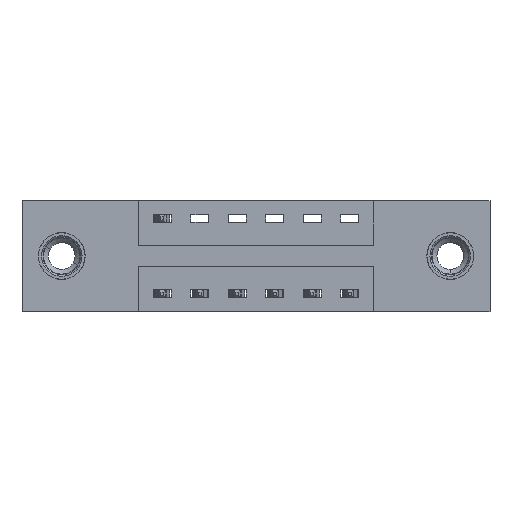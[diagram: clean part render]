
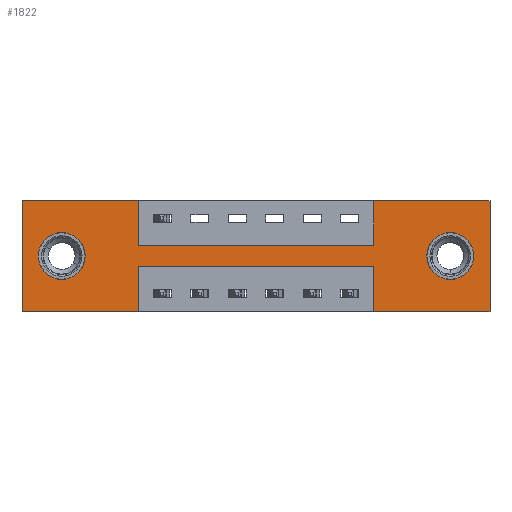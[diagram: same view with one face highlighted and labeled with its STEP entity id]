
A CAD part, front view. The second image highlights one B-rep face of the part: STEP entity #1822.
In plain terms, the highlighted planar face has unit normal (0, -1, 0).
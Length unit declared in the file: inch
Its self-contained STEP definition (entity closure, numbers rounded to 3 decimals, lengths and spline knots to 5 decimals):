
#137 = EDGE_CURVE ( 'NONE', #8113, #5049, #6763, .T. ) ;
#232 = DIRECTION ( 'NONE',  ( 0., 1., 0. ) ) ;
#270 = FACE_BOUND ( 'NONE', #4870, .T. ) ;
#615 = CARTESIAN_POINT ( 'NONE',  ( 0.3875, 0., 0. ) ) ;
#638 = EDGE_CURVE ( 'NONE', #8432, #5361, #3279, .T. ) ;
#784 = CIRCLE ( 'NONE', #4674, 0.078 ) ;
#791 = CARTESIAN_POINT ( 'NONE',  ( 0., 0., 0. ) ) ;
#846 = VERTEX_POINT ( 'NONE', #2154 ) ;
#847 = ORIENTED_EDGE ( 'NONE', *, *, #6527, .T. ) ;
#1048 = EDGE_CURVE ( 'NONE', #5049, #8432, #7312, .T. ) ;
#1092 = CARTESIAN_POINT ( 'NONE',  ( 1.1725, 0., -0.37 ) ) ;
#1111 = CARTESIAN_POINT ( 'NONE',  ( 0.1325, 0., -0.263 ) ) ;
#1154 = EDGE_CURVE ( 'NONE', #3479, #5919, #2931, .T. ) ;
#1217 = LINE ( 'NONE', #3399, #6909 ) ;
#1261 = VECTOR ( 'NONE', #5626, 39.37008 ) ;
#1312 = ORIENTED_EDGE ( 'NONE', *, *, #8654, .F. ) ;
#1360 = ORIENTED_EDGE ( 'NONE', *, *, #6315, .F. ) ;
#1410 = CARTESIAN_POINT ( 'NONE',  ( 0., 0., -0.37 ) ) ;
#1444 = ORIENTED_EDGE ( 'NONE', *, *, #6702, .T. ) ;
#1599 = CARTESIAN_POINT ( 'NONE',  ( 0.1325, 0., -0.185 ) ) ;
#1620 = ORIENTED_EDGE ( 'NONE', *, *, #5945, .T. ) ;
#1822 = ADVANCED_FACE ( 'NONE', ( #270, #4284, #8024 ), #6046, .T. ) ;
#2034 = AXIS2_PLACEMENT_3D ( 'NONE', #6021, #5985, #5983 ) ;
#2154 = CARTESIAN_POINT ( 'NONE',  ( 0.1325, 0., -0.107 ) ) ;
#2155 = CARTESIAN_POINT ( 'NONE',  ( 1.1725, 0., -0.37 ) ) ;
#2287 = LINE ( 'NONE', #4953, #6199 ) ;
#2290 = EDGE_CURVE ( 'NONE', #6367, #3479, #6001, .T. ) ;
#2329 = EDGE_CURVE ( 'NONE', #5919, #8113, #5535, .T. ) ;
#2351 = DIRECTION ( 'NONE',  ( 0., 0., 1. ) ) ;
#2364 = CARTESIAN_POINT ( 'NONE',  ( 1.4275, 0., -0.185 ) ) ;
#2379 = CARTESIAN_POINT ( 'NONE',  ( 0.3875, 0., -0.22 ) ) ;
#2402 = CARTESIAN_POINT ( 'NONE',  ( 1.1725, 0., 0. ) ) ;
#2438 = AXIS2_PLACEMENT_3D ( 'NONE', #7501, #3096, #8303 ) ;
#2605 = ORIENTED_EDGE ( 'NONE', *, *, #1048, .F. ) ;
#2648 = VERTEX_POINT ( 'NONE', #2155 ) ;
#2654 = CARTESIAN_POINT ( 'NONE',  ( 1.4275, 0., -0.107 ) ) ;
#2705 = VECTOR ( 'NONE', #3577, 39.37008 ) ;
#2770 = CARTESIAN_POINT ( 'NONE',  ( 0.3875, 0., -0.15 ) ) ;
#2895 = VERTEX_POINT ( 'NONE', #1111 ) ;
#2931 = LINE ( 'NONE', #9127, #6603 ) ;
#2957 = ORIENTED_EDGE ( 'NONE', *, *, #2290, .F. ) ;
#3096 = DIRECTION ( 'NONE',  ( 0., 1., 0. ) ) ;
#3137 = DIRECTION ( 'NONE',  ( 0., 0., -1. ) ) ;
#3279 = LINE ( 'NONE', #5663, #1261 ) ;
#3356 = CARTESIAN_POINT ( 'NONE',  ( 1.1725, 0., -0.15 ) ) ;
#3399 = CARTESIAN_POINT ( 'NONE',  ( 0., 0., -0.37 ) ) ;
#3479 = VERTEX_POINT ( 'NONE', #791 ) ;
#3577 = DIRECTION ( 'NONE',  ( 0., 0., -1. ) ) ;
#3591 = ORIENTED_EDGE ( 'NONE', *, *, #2329, .F. ) ;
#3606 = ORIENTED_EDGE ( 'NONE', *, *, #6813, .F. ) ;
#3710 = LINE ( 'NONE', #7843, #7627 ) ;
#3767 = LINE ( 'NONE', #9277, #9531 ) ;
#3827 = DIRECTION ( 'NONE',  ( 0., 0., -1. ) ) ;
#3830 = VECTOR ( 'NONE', #3827, 39.37008 ) ;
#3847 = CARTESIAN_POINT ( 'NONE',  ( 0.3875, 0., 0. ) ) ;
#4049 = DIRECTION ( 'NONE',  ( 0., 0., 1. ) ) ;
#4052 = VECTOR ( 'NONE', #4049, 39.37008 ) ;
#4063 = CARTESIAN_POINT ( 'NONE',  ( 0.3875, 0., -0.15 ) ) ;
#4096 = CARTESIAN_POINT ( 'NONE',  ( 0., 0., 0. ) ) ;
#4133 = DIRECTION ( 'NONE',  ( -1., 0., 0. ) ) ;
#4202 = ORIENTED_EDGE ( 'NONE', *, *, #9693, .F. ) ;
#4284 = FACE_BOUND ( 'NONE', #9360, .T. ) ;
#4380 = CIRCLE ( 'NONE', #7654, 0.078 ) ;
#4461 = CARTESIAN_POINT ( 'NONE',  ( 1.1725, 0., -0.22 ) ) ;
#4574 = VECTOR ( 'NONE', #9373, 39.37008 ) ;
#4666 = LINE ( 'NONE', #8022, #2705 ) ;
#4674 = AXIS2_PLACEMENT_3D ( 'NONE', #2364, #7536, #3137 ) ;
#4747 = CARTESIAN_POINT ( 'NONE',  ( 1.4275, 0., -0.185 ) ) ;
#4870 = EDGE_LOOP ( 'NONE', ( #1444, #847 ) ) ;
#4953 = CARTESIAN_POINT ( 'NONE',  ( 0.3875, 0., -0.22 ) ) ;
#5049 = VERTEX_POINT ( 'NONE', #3356 ) ;
#5342 = VECTOR ( 'NONE', #9519, 39.37008 ) ;
#5361 = VERTEX_POINT ( 'NONE', #5916 ) ;
#5489 = DIRECTION ( 'NONE',  ( 0., 0., -1. ) ) ;
#5535 = LINE ( 'NONE', #3847, #3830 ) ;
#5540 = DIRECTION ( 'NONE',  ( -1., 0., 0. ) ) ;
#5541 = DIRECTION ( 'NONE',  ( 0., 0., 1. ) ) ;
#5561 = ORIENTED_EDGE ( 'NONE', *, *, #7461, .F. ) ;
#5589 = ORIENTED_EDGE ( 'NONE', *, *, #137, .F. ) ;
#5626 = DIRECTION ( 'NONE',  ( 1., 0., 0. ) ) ;
#5661 = CARTESIAN_POINT ( 'NONE',  ( 1.56, 0., -0.37 ) ) ;
#5663 = CARTESIAN_POINT ( 'NONE',  ( 0., 0., 0. ) ) ;
#5916 = CARTESIAN_POINT ( 'NONE',  ( 1.56, 0., 0. ) ) ;
#5919 = VERTEX_POINT ( 'NONE', #615 ) ;
#5934 = CIRCLE ( 'NONE', #2438, 0.078 ) ;
#5945 = EDGE_CURVE ( 'NONE', #2895, #846, #5934, .T. ) ;
#5975 = VERTEX_POINT ( 'NONE', #8336 ) ;
#5983 = DIRECTION ( 'NONE',  ( 0., 0., -1. ) ) ;
#5985 = DIRECTION ( 'NONE',  ( 0., -1., 0. ) ) ;
#6001 = LINE ( 'NONE', #4096, #4052 ) ;
#6006 = ORIENTED_EDGE ( 'NONE', *, *, #9070, .T. ) ;
#6021 = CARTESIAN_POINT ( 'NONE',  ( 0., 0., -0.37 ) ) ;
#6046 = PLANE ( 'NONE',  #2034 ) ;
#6199 = VECTOR ( 'NONE', #9513, 39.37008 ) ;
#6201 = DIRECTION ( 'NONE',  ( 0., 0., -1. ) ) ;
#6287 = VECTOR ( 'NONE', #5541, 39.37008 ) ;
#6315 = EDGE_CURVE ( 'NONE', #7762, #5975, #4666, .T. ) ;
#6367 = VERTEX_POINT ( 'NONE', #1410 ) ;
#6464 = VERTEX_POINT ( 'NONE', #4461 ) ;
#6527 = EDGE_CURVE ( 'NONE', #7573, #9227, #784, .T. ) ;
#6603 = VECTOR ( 'NONE', #9144, 39.37008 ) ;
#6650 = ORIENTED_EDGE ( 'NONE', *, *, #1154, .F. ) ;
#6702 = EDGE_CURVE ( 'NONE', #9227, #7573, #4380, .T. ) ;
#6763 = LINE ( 'NONE', #4063, #4574 ) ;
#6770 = LINE ( 'NONE', #1092, #6287 ) ;
#6773 = DIRECTION ( 'NONE',  ( 0., 1., 0. ) ) ;
#6813 = EDGE_CURVE ( 'NONE', #5975, #6367, #3710, .T. ) ;
#6845 = EDGE_LOOP ( 'NONE', ( #1360, #5561, #1312, #7402, #4202, #8854, #2605, #5589, #3591, #6650, #2957, #3606 ) ) ;
#6909 = VECTOR ( 'NONE', #4133, 39.37008 ) ;
#7312 = LINE ( 'NONE', #9595, #5342 ) ;
#7371 = EDGE_CURVE ( 'NONE', #9270, #2648, #1217, .T. ) ;
#7402 = ORIENTED_EDGE ( 'NONE', *, *, #7371, .F. ) ;
#7461 = EDGE_CURVE ( 'NONE', #6464, #7762, #2287, .T. ) ;
#7485 = AXIS2_PLACEMENT_3D ( 'NONE', #1599, #6773, #2351 ) ;
#7501 = CARTESIAN_POINT ( 'NONE',  ( 0.1325, 0., -0.185 ) ) ;
#7536 = DIRECTION ( 'NONE',  ( 0., 1., 0. ) ) ;
#7573 = VERTEX_POINT ( 'NONE', #8911 ) ;
#7627 = VECTOR ( 'NONE', #5540, 39.37008 ) ;
#7654 = AXIS2_PLACEMENT_3D ( 'NONE', #4747, #232, #5489 ) ;
#7762 = VERTEX_POINT ( 'NONE', #2379 ) ;
#7843 = CARTESIAN_POINT ( 'NONE',  ( 0., 0., -0.37 ) ) ;
#8022 = CARTESIAN_POINT ( 'NONE',  ( 0.3875, 0., -0.37 ) ) ;
#8024 = FACE_OUTER_BOUND ( 'NONE', #6845, .T. ) ;
#8113 = VERTEX_POINT ( 'NONE', #2770 ) ;
#8303 = DIRECTION ( 'NONE',  ( 0., 0., 1. ) ) ;
#8331 = CIRCLE ( 'NONE', #7485, 0.078 ) ;
#8336 = CARTESIAN_POINT ( 'NONE',  ( 0.3875, 0., -0.37 ) ) ;
#8432 = VERTEX_POINT ( 'NONE', #2402 ) ;
#8654 = EDGE_CURVE ( 'NONE', #2648, #6464, #6770, .T. ) ;
#8854 = ORIENTED_EDGE ( 'NONE', *, *, #638, .F. ) ;
#8911 = CARTESIAN_POINT ( 'NONE',  ( 1.4275, 0., -0.263 ) ) ;
#9070 = EDGE_CURVE ( 'NONE', #846, #2895, #8331, .T. ) ;
#9127 = CARTESIAN_POINT ( 'NONE',  ( 0., 0., 0. ) ) ;
#9144 = DIRECTION ( 'NONE',  ( 1., 0., 0. ) ) ;
#9227 = VERTEX_POINT ( 'NONE', #2654 ) ;
#9270 = VERTEX_POINT ( 'NONE', #5661 ) ;
#9277 = CARTESIAN_POINT ( 'NONE',  ( 1.56, 0., 0. ) ) ;
#9360 = EDGE_LOOP ( 'NONE', ( #6006, #1620 ) ) ;
#9373 = DIRECTION ( 'NONE',  ( 1., 0., 0. ) ) ;
#9513 = DIRECTION ( 'NONE',  ( -1., 0., 0. ) ) ;
#9519 = DIRECTION ( 'NONE',  ( 0., 0., 1. ) ) ;
#9531 = VECTOR ( 'NONE', #6201, 39.37008 ) ;
#9595 = CARTESIAN_POINT ( 'NONE',  ( 1.1725, 0., 0. ) ) ;
#9693 = EDGE_CURVE ( 'NONE', #5361, #9270, #3767, .T. ) ;
